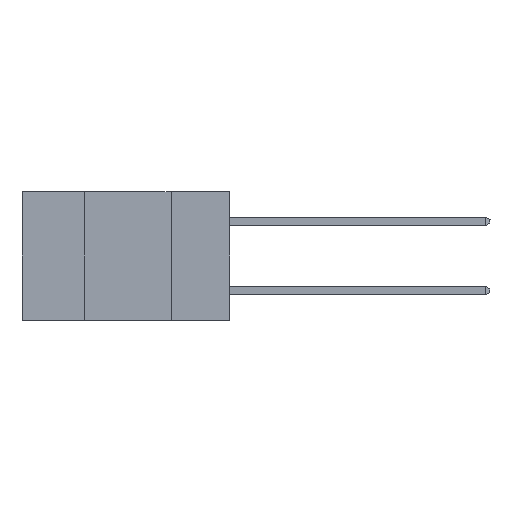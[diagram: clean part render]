
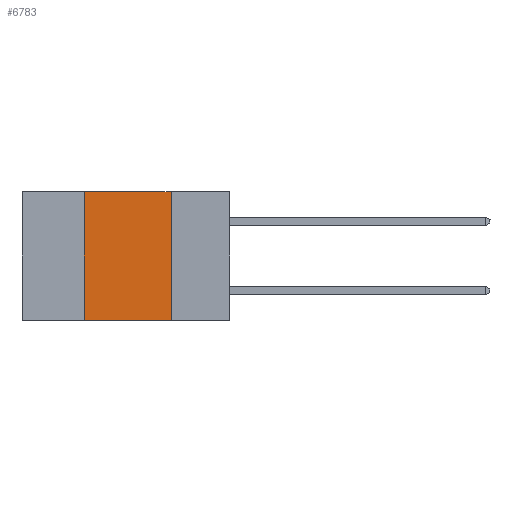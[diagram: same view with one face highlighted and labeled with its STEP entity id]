
A CAD part, left-side view. The second image highlights one B-rep face of the part: STEP entity #6783.
In plain terms, the highlighted planar face has unit normal (-1, 0, 0).
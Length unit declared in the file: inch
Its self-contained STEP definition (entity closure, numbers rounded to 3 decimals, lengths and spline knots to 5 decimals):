
#30 = LINE ( 'NONE', #3668, #10934 ) ;
#857 = EDGE_CURVE ( 'NONE', #6940, #9286, #1856, .T. ) ;
#1166 = DIRECTION ( 'NONE',  ( 0., 0., 1. ) ) ;
#1614 = ORIENTED_EDGE ( 'NONE', *, *, #9007, .F. ) ;
#1628 = CARTESIAN_POINT ( 'NONE',  ( 0., 0.42, 0. ) ) ;
#1656 = CARTESIAN_POINT ( 'NONE',  ( 0., 0.17, -0.37 ) ) ;
#1856 = LINE ( 'NONE', #6426, #6447 ) ;
#1899 = VECTOR ( 'NONE', #11472, 39.37008 ) ;
#2177 = ORIENTED_EDGE ( 'NONE', *, *, #2700, .F. ) ;
#2700 = EDGE_CURVE ( 'NONE', #11420, #9948, #11360, .T. ) ;
#3235 = ORIENTED_EDGE ( 'NONE', *, *, #11063, .F. ) ;
#3668 = CARTESIAN_POINT ( 'NONE',  ( 0., 0.42, -0.37 ) ) ;
#3729 = LINE ( 'NONE', #10812, #5438 ) ;
#5438 = VECTOR ( 'NONE', #8975, 39.37008 ) ;
#5499 = DIRECTION ( 'NONE',  ( 0., -1., 0. ) ) ;
#6102 = FACE_OUTER_BOUND ( 'NONE', #9428, .T. ) ;
#6426 = CARTESIAN_POINT ( 'NONE',  ( 0., 0.6, -0.37 ) ) ;
#6447 = VECTOR ( 'NONE', #5499, 39.37008 ) ;
#6783 = ADVANCED_FACE ( 'NONE', ( #6102 ), #11629, .F. ) ;
#6849 = CARTESIAN_POINT ( 'NONE',  ( 0., 0.42, -0.37 ) ) ;
#6940 = VERTEX_POINT ( 'NONE', #6849 ) ;
#7167 = ORIENTED_EDGE ( 'NONE', *, *, #857, .T. ) ;
#7347 = DIRECTION ( 'NONE',  ( 1., 0., 0. ) ) ;
#7562 = DIRECTION ( 'NONE',  ( 0., 0., -1. ) ) ;
#7751 = CARTESIAN_POINT ( 'NONE',  ( 0., 0.17, 0. ) ) ;
#8228 = AXIS2_PLACEMENT_3D ( 'NONE', #8835, #7347, #7562 ) ;
#8835 = CARTESIAN_POINT ( 'NONE',  ( 0., 0.6, 0. ) ) ;
#8975 = DIRECTION ( 'NONE',  ( 0., 0., -1. ) ) ;
#9007 = EDGE_CURVE ( 'NONE', #9948, #9286, #3729, .T. ) ;
#9286 = VERTEX_POINT ( 'NONE', #1656 ) ;
#9428 = EDGE_LOOP ( 'NONE', ( #1614, #2177, #3235, #7167 ) ) ;
#9518 = CARTESIAN_POINT ( 'NONE',  ( 0., 0.6, 0. ) ) ;
#9948 = VERTEX_POINT ( 'NONE', #7751 ) ;
#10812 = CARTESIAN_POINT ( 'NONE',  ( 0., 0.17, -0.37 ) ) ;
#10934 = VECTOR ( 'NONE', #1166, 39.37008 ) ;
#11063 = EDGE_CURVE ( 'NONE', #6940, #11420, #30, .T. ) ;
#11360 = LINE ( 'NONE', #9518, #1899 ) ;
#11420 = VERTEX_POINT ( 'NONE', #1628 ) ;
#11472 = DIRECTION ( 'NONE',  ( 0., -1., 0. ) ) ;
#11629 = PLANE ( 'NONE',  #8228 ) ;
